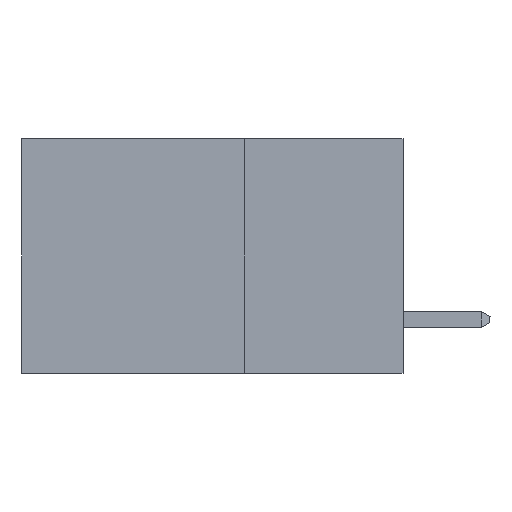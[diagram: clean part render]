
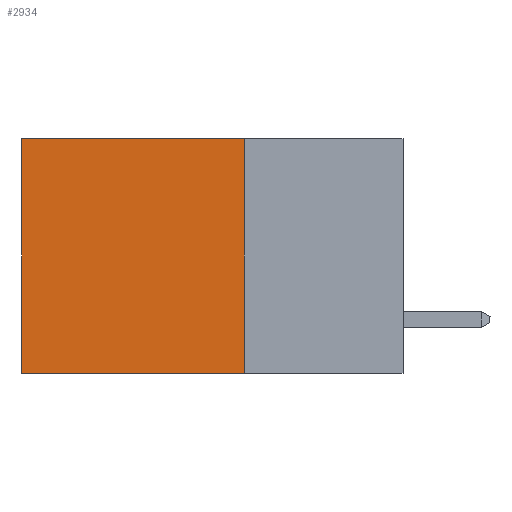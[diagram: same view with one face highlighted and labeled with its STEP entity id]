
A CAD part, left-side view. The second image highlights one B-rep face of the part: STEP entity #2934.
In plain terms, the highlighted planar face has unit normal (-1, 0, 0).
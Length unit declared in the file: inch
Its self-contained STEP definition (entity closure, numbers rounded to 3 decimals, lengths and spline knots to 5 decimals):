
#1482 = VECTOR ( 'NONE', #20421, 39.37008 ) ;
#2234 = EDGE_LOOP ( 'NONE', ( #16144, #33029, #43060, #47474 ) ) ;
#2934 = ADVANCED_FACE ( 'NONE', ( #45662 ), #41838, .F. ) ;
#6004 = CARTESIAN_POINT ( 'NONE',  ( 0.2875, 0.25, 0. ) ) ;
#7046 = CARTESIAN_POINT ( 'NONE',  ( 0.2875, 0.25, 0. ) ) ;
#12364 = EDGE_CURVE ( 'NONE', #43363, #13955, #34743, .T. ) ;
#13434 = LINE ( 'NONE', #27871, #1482 ) ;
#13955 = VERTEX_POINT ( 'NONE', #14782 ) ;
#14128 = VERTEX_POINT ( 'NONE', #38550 ) ;
#14782 = CARTESIAN_POINT ( 'NONE',  ( 0.2875, 0.25, -0.37 ) ) ;
#14912 = AXIS2_PLACEMENT_3D ( 'NONE', #38467, #46141, #16836 ) ;
#16144 = ORIENTED_EDGE ( 'NONE', *, *, #41192, .T. ) ;
#16836 = DIRECTION ( 'NONE',  ( 0., 0., -1. ) ) ;
#19387 = CARTESIAN_POINT ( 'NONE',  ( 0.2875, 0.25, 0. ) ) ;
#20421 = DIRECTION ( 'NONE',  ( 0., 1., 0. ) ) ;
#21450 = VECTOR ( 'NONE', #45554, 39.37008 ) ;
#25520 = CARTESIAN_POINT ( 'NONE',  ( 0.2875, 0.6, -0.37 ) ) ;
#26222 = EDGE_CURVE ( 'NONE', #13955, #31438, #13434, .T. ) ;
#26808 = LINE ( 'NONE', #27280, #43807 ) ;
#27280 = CARTESIAN_POINT ( 'NONE',  ( 0.2875, 0.6, 0. ) ) ;
#27505 = VECTOR ( 'NONE', #43558, 39.37008 ) ;
#27871 = CARTESIAN_POINT ( 'NONE',  ( 0.2875, 0.25, -0.37 ) ) ;
#28659 = LINE ( 'NONE', #7046, #27505 ) ;
#31438 = VERTEX_POINT ( 'NONE', #25520 ) ;
#33029 = ORIENTED_EDGE ( 'NONE', *, *, #26222, .F. ) ;
#34743 = LINE ( 'NONE', #19387, #21450 ) ;
#35909 = EDGE_CURVE ( 'NONE', #43363, #14128, #28659, .T. ) ;
#38467 = CARTESIAN_POINT ( 'NONE',  ( 0.2875, 0.25, 0. ) ) ;
#38550 = CARTESIAN_POINT ( 'NONE',  ( 0.2875, 0.6, 0. ) ) ;
#41192 = EDGE_CURVE ( 'NONE', #14128, #31438, #26808, .T. ) ;
#41467 = DIRECTION ( 'NONE',  ( 0., 0., -1. ) ) ;
#41838 = PLANE ( 'NONE',  #14912 ) ;
#43060 = ORIENTED_EDGE ( 'NONE', *, *, #12364, .F. ) ;
#43363 = VERTEX_POINT ( 'NONE', #6004 ) ;
#43558 = DIRECTION ( 'NONE',  ( 0., 1., 0. ) ) ;
#43807 = VECTOR ( 'NONE', #41467, 39.37008 ) ;
#45554 = DIRECTION ( 'NONE',  ( 0., 0., -1. ) ) ;
#45662 = FACE_OUTER_BOUND ( 'NONE', #2234, .T. ) ;
#46141 = DIRECTION ( 'NONE',  ( 1., 0., 0. ) ) ;
#47474 = ORIENTED_EDGE ( 'NONE', *, *, #35909, .T. ) ;
